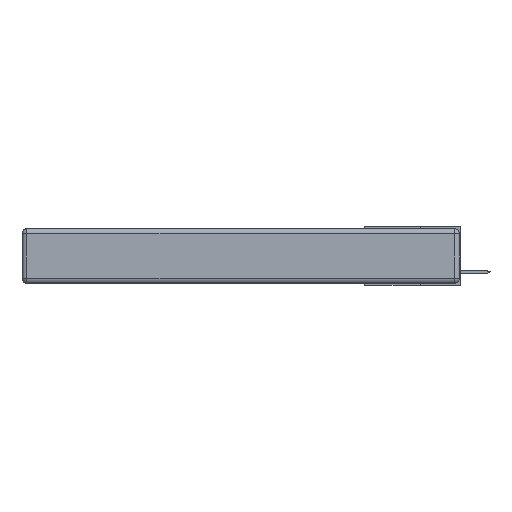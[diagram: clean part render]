
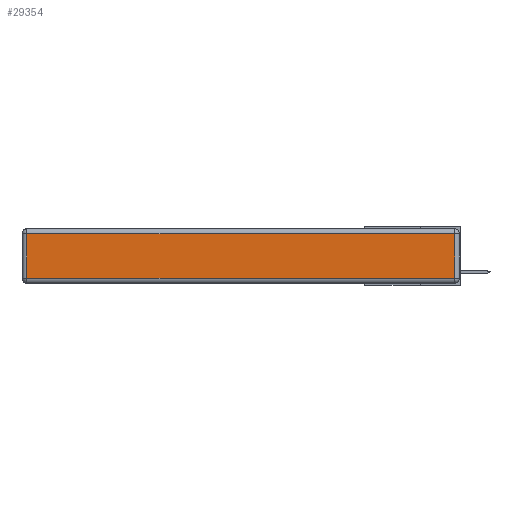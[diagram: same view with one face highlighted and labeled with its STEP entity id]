
A CAD part, left-side view. The second image highlights one B-rep face of the part: STEP entity #29354.
In plain terms, the highlighted planar face has unit normal (-1, 0, 0).
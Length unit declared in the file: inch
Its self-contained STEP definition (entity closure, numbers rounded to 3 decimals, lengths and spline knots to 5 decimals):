
#148 = VECTOR ( 'NONE', #3308, 39.37008 ) ;
#1488 = DIRECTION ( 'NONE',  ( 0., 0., 1. ) ) ;
#2437 = CARTESIAN_POINT ( 'NONE',  ( 0., 2.75, -0.03 ) ) ;
#2977 = DIRECTION ( 'NONE',  ( 0., 0., -1. ) ) ;
#3308 = DIRECTION ( 'NONE',  ( 0., 1., 0. ) ) ;
#3642 = CARTESIAN_POINT ( 'NONE',  ( 0., 0.03, -0.343 ) ) ;
#3778 = CARTESIAN_POINT ( 'NONE',  ( 0., 0.03, -0.313 ) ) ;
#3969 = PLANE ( 'NONE',  #11327 ) ;
#4246 = CARTESIAN_POINT ( 'NONE',  ( 0., 2.72, -0.03 ) ) ;
#6334 = ORIENTED_EDGE ( 'NONE', *, *, #13636, .T. ) ;
#7022 = VERTEX_POINT ( 'NONE', #23981 ) ;
#7878 = LINE ( 'NONE', #22575, #25937 ) ;
#8091 = ORIENTED_EDGE ( 'NONE', *, *, #17113, .T. ) ;
#11327 = AXIS2_PLACEMENT_3D ( 'NONE', #15224, #25780, #28364 ) ;
#12279 = LINE ( 'NONE', #3642, #24081 ) ;
#13635 = EDGE_CURVE ( 'NONE', #22768, #17894, #12279, .T. ) ;
#13636 = EDGE_CURVE ( 'NONE', #7022, #22768, #7878, .T. ) ;
#14465 = CARTESIAN_POINT ( 'NONE',  ( 0., 2.72, -0.343 ) ) ;
#15224 = CARTESIAN_POINT ( 'NONE',  ( 0., 0., -0.343 ) ) ;
#17113 = EDGE_CURVE ( 'NONE', #17894, #18639, #20278, .T. ) ;
#17894 = VERTEX_POINT ( 'NONE', #23480 ) ;
#18639 = VERTEX_POINT ( 'NONE', #4246 ) ;
#20278 = LINE ( 'NONE', #2437, #148 ) ;
#20849 = LINE ( 'NONE', #14465, #23814 ) ;
#22575 = CARTESIAN_POINT ( 'NONE',  ( 0., 0., -0.313 ) ) ;
#22768 = VERTEX_POINT ( 'NONE', #3778 ) ;
#23480 = CARTESIAN_POINT ( 'NONE',  ( 0., 0.03, -0.03 ) ) ;
#23814 = VECTOR ( 'NONE', #2977, 39.37008 ) ;
#23921 = EDGE_LOOP ( 'NONE', ( #6334, #30076, #8091, #27809 ) ) ;
#23981 = CARTESIAN_POINT ( 'NONE',  ( 0., 2.72, -0.313 ) ) ;
#24081 = VECTOR ( 'NONE', #1488, 39.37008 ) ;
#24862 = EDGE_CURVE ( 'NONE', #18639, #7022, #20849, .T. ) ;
#25780 = DIRECTION ( 'NONE',  ( -1., 0., 0. ) ) ;
#25937 = VECTOR ( 'NONE', #27446, 39.37008 ) ;
#26826 = FACE_OUTER_BOUND ( 'NONE', #23921, .T. ) ;
#27446 = DIRECTION ( 'NONE',  ( 0., -1., 0. ) ) ;
#27809 = ORIENTED_EDGE ( 'NONE', *, *, #24862, .T. ) ;
#28364 = DIRECTION ( 'NONE',  ( 0., 0., 1. ) ) ;
#29354 = ADVANCED_FACE ( 'NONE', ( #26826 ), #3969, .T. ) ;
#30076 = ORIENTED_EDGE ( 'NONE', *, *, #13635, .T. ) ;
